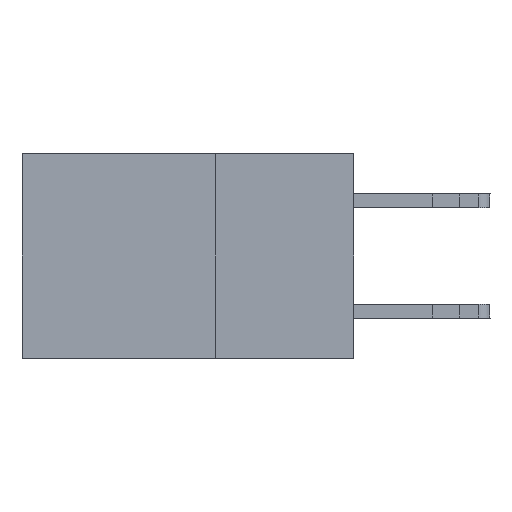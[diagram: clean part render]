
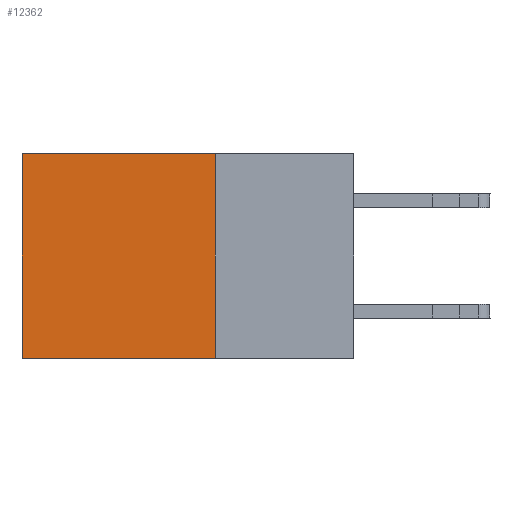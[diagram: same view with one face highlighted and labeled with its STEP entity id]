
A CAD part, left-side view. The second image highlights one B-rep face of the part: STEP entity #12362.
In plain terms, the highlighted planar face has unit normal (-1, 0, 0).
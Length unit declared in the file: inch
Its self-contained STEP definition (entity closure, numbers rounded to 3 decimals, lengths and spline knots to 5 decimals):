
#844 = LINE ( 'NONE', #5752, #8547 ) ;
#1242 = LINE ( 'NONE', #1858, #9792 ) ;
#1450 = DIRECTION ( 'NONE',  ( 0., 0., -1. ) ) ;
#1655 = CARTESIAN_POINT ( 'NONE',  ( 0.2875, 0.25, 0. ) ) ;
#1787 = CARTESIAN_POINT ( 'NONE',  ( 0.2875, 0.6, -0.37 ) ) ;
#1858 = CARTESIAN_POINT ( 'NONE',  ( 0.2875, 0.6, 0. ) ) ;
#2167 = ORIENTED_EDGE ( 'NONE', *, *, #10189, .T. ) ;
#2633 = CARTESIAN_POINT ( 'NONE',  ( 0.2875, 0.25, 0. ) ) ;
#2802 = VERTEX_POINT ( 'NONE', #13154 ) ;
#2908 = CARTESIAN_POINT ( 'NONE',  ( 0.2875, 0.25, 0. ) ) ;
#3015 = DIRECTION ( 'NONE',  ( 0., 1., 0. ) ) ;
#3595 = LINE ( 'NONE', #1655, #7991 ) ;
#3695 = DIRECTION ( 'NONE',  ( 0., 0., -1. ) ) ;
#4794 = EDGE_CURVE ( 'NONE', #13070, #9089, #10214, .T. ) ;
#4958 = ORIENTED_EDGE ( 'NONE', *, *, #4794, .F. ) ;
#5435 = ORIENTED_EDGE ( 'NONE', *, *, #7770, .T. ) ;
#5752 = CARTESIAN_POINT ( 'NONE',  ( 0.2875, 0.25, -0.37 ) ) ;
#6540 = DIRECTION ( 'NONE',  ( 1., 0., 0. ) ) ;
#7770 = EDGE_CURVE ( 'NONE', #13070, #2802, #3595, .T. ) ;
#7991 = VECTOR ( 'NONE', #3015, 39.37008 ) ;
#8547 = VECTOR ( 'NONE', #11276, 39.37008 ) ;
#8701 = DIRECTION ( 'NONE',  ( 0., 0., -1. ) ) ;
#9089 = VERTEX_POINT ( 'NONE', #15247 ) ;
#9746 = VECTOR ( 'NONE', #3695, 39.37008 ) ;
#9792 = VECTOR ( 'NONE', #8701, 39.37008 ) ;
#10189 = EDGE_CURVE ( 'NONE', #2802, #16146, #1242, .T. ) ;
#10214 = LINE ( 'NONE', #15393, #9746 ) ;
#11276 = DIRECTION ( 'NONE',  ( 0., 1., 0. ) ) ;
#12020 = PLANE ( 'NONE',  #16123 ) ;
#12362 = ADVANCED_FACE ( 'NONE', ( #12558 ), #12020, .F. ) ;
#12558 = FACE_OUTER_BOUND ( 'NONE', #13126, .T. ) ;
#13070 = VERTEX_POINT ( 'NONE', #2908 ) ;
#13126 = EDGE_LOOP ( 'NONE', ( #2167, #15538, #4958, #5435 ) ) ;
#13154 = CARTESIAN_POINT ( 'NONE',  ( 0.2875, 0.6, 0. ) ) ;
#13226 = EDGE_CURVE ( 'NONE', #9089, #16146, #844, .T. ) ;
#15247 = CARTESIAN_POINT ( 'NONE',  ( 0.2875, 0.25, -0.37 ) ) ;
#15393 = CARTESIAN_POINT ( 'NONE',  ( 0.2875, 0.25, 0. ) ) ;
#15538 = ORIENTED_EDGE ( 'NONE', *, *, #13226, .F. ) ;
#16123 = AXIS2_PLACEMENT_3D ( 'NONE', #2633, #6540, #1450 ) ;
#16146 = VERTEX_POINT ( 'NONE', #1787 ) ;
